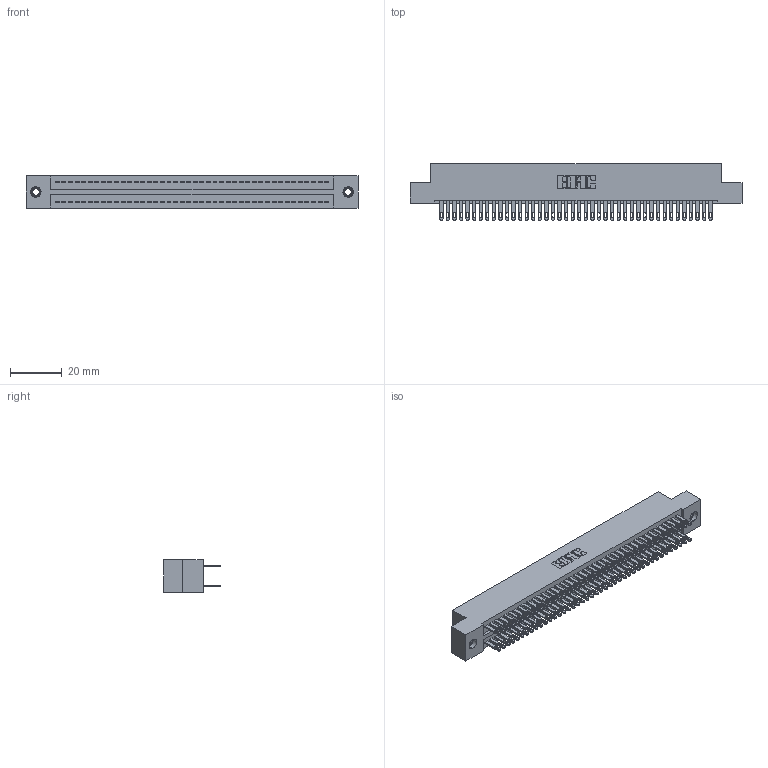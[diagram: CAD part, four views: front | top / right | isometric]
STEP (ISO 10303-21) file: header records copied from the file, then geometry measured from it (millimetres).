
FILE_DESCRIPTION (( 'STEP AP203' ), '1' );
FILE_NAME ('325-084-500-207.STEP', '2020-02-25T04:58:23', ( '' ), ( '' ), 'SwSTEP 2.0', 'SolidWorks 2016', '' );
FILE_SCHEMA (( 'CONFIG_CONTROL_DESIGN' ));
Length unit declared in the file: inch
Products named in the file (4): 325-292-001_325-293-100; 325 Part_TI; 325-084-500-207; 345-250-001_345-250-005-103
Assembly tree (87 placements, depth 2):
  325-084-500-207
    325 Part_TI
    325-292-001_325-293-100  x84
    345-250-001_345-250-005-103  x2
Bounding box: 128.4 x 21.84 x 12.45 mm (x, y, z)
Volume: 16818.7 mm3; surface area: 21261.3 mm2
Topology: 87 solids, 87 shells, 4206 faces, 12795 edges, 8522 vertices
Faces by surface type: plane 2622, cylinder 1568, cone 12, torus 4
Entity records: 28136 total; most frequent: CARTESIAN_POINT 4645, ORIENTED_EDGE 4574, DIRECTION 4001, EDGE_CURVE 2287, LINE 2135, VECTOR 2135, VERTEX_POINT 1520, AXIS2_PLACEMENT_3D 933
